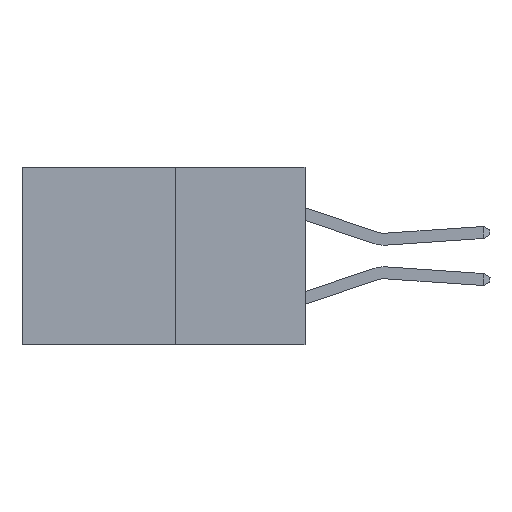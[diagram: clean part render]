
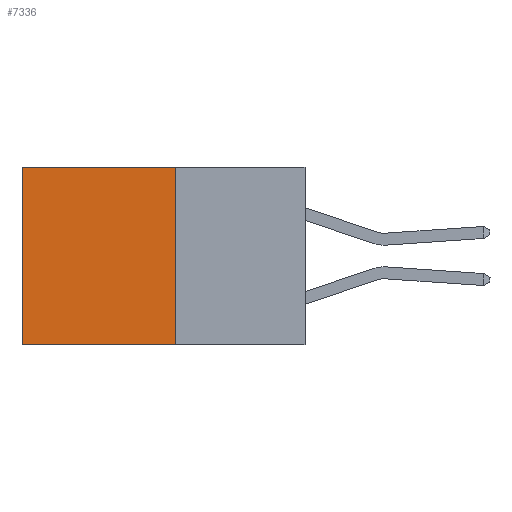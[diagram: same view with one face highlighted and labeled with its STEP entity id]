
A CAD part, left-side view. The second image highlights one B-rep face of the part: STEP entity #7336.
In plain terms, the highlighted planar face has unit normal (-1, 0, 0).
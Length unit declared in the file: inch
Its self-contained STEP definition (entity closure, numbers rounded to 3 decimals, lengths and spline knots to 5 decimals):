
#1226 = EDGE_CURVE ( 'NONE', #4120, #15857, #4964, .T. ) ;
#2653 = FACE_OUTER_BOUND ( 'NONE', #14491, .T. ) ;
#3341 = CARTESIAN_POINT ( 'NONE',  ( 0.277, 0.59, -0.37 ) ) ;
#3538 = CARTESIAN_POINT ( 'NONE',  ( 0.277, 0.27, -0.37 ) ) ;
#4120 = VERTEX_POINT ( 'NONE', #21386 ) ;
#4964 = LINE ( 'NONE', #3341, #13971 ) ;
#5347 = DIRECTION ( 'NONE',  ( 0., 0., -1. ) ) ;
#5395 = ORIENTED_EDGE ( 'NONE', *, *, #21668, .T. ) ;
#5653 = CARTESIAN_POINT ( 'NONE',  ( 0.277, 0.27, -0.37 ) ) ;
#6136 = CARTESIAN_POINT ( 'NONE',  ( 0.277, 0.27, -0.37 ) ) ;
#7336 = ADVANCED_FACE ( 'NONE', ( #2653 ), #21243, .F. ) ;
#9477 = CARTESIAN_POINT ( 'NONE',  ( 0.277, 0.27, -0.37 ) ) ;
#10611 = ORIENTED_EDGE ( 'NONE', *, *, #1226, .T. ) ;
#11216 = AXIS2_PLACEMENT_3D ( 'NONE', #3538, #16066, #5347 ) ;
#13971 = VECTOR ( 'NONE', #18810, 39.37008 ) ;
#14081 = CARTESIAN_POINT ( 'NONE',  ( 0.277, 0.27, 0. ) ) ;
#14491 = EDGE_LOOP ( 'NONE', ( #10611, #14685, #21792, #5395 ) ) ;
#14685 = ORIENTED_EDGE ( 'NONE', *, *, #15183, .F. ) ;
#14712 = EDGE_CURVE ( 'NONE', #16545, #15268, #15912, .T. ) ;
#15183 = EDGE_CURVE ( 'NONE', #15268, #15857, #19981, .T. ) ;
#15268 = VERTEX_POINT ( 'NONE', #9477 ) ;
#15366 = VECTOR ( 'NONE', #20319, 39.37008 ) ;
#15391 = VECTOR ( 'NONE', #22630, 39.37008 ) ;
#15857 = VERTEX_POINT ( 'NONE', #16239 ) ;
#15912 = LINE ( 'NONE', #6136, #15366 ) ;
#16066 = DIRECTION ( 'NONE',  ( 1., 0., 0. ) ) ;
#16239 = CARTESIAN_POINT ( 'NONE',  ( 0.277, 0.59, -0.37 ) ) ;
#16545 = VERTEX_POINT ( 'NONE', #14081 ) ;
#18810 = DIRECTION ( 'NONE',  ( 0., 0., -1. ) ) ;
#19443 = VECTOR ( 'NONE', #19856, 39.37008 ) ;
#19488 = LINE ( 'NONE', #20899, #15391 ) ;
#19856 = DIRECTION ( 'NONE',  ( 0., 1., 0. ) ) ;
#19981 = LINE ( 'NONE', #5653, #19443 ) ;
#20319 = DIRECTION ( 'NONE',  ( 0., 0., -1. ) ) ;
#20899 = CARTESIAN_POINT ( 'NONE',  ( 0.277, 0.27, 0. ) ) ;
#21243 = PLANE ( 'NONE',  #11216 ) ;
#21386 = CARTESIAN_POINT ( 'NONE',  ( 0.277, 0.59, 0. ) ) ;
#21668 = EDGE_CURVE ( 'NONE', #16545, #4120, #19488, .T. ) ;
#21792 = ORIENTED_EDGE ( 'NONE', *, *, #14712, .F. ) ;
#22630 = DIRECTION ( 'NONE',  ( 0., 1., 0. ) ) ;
